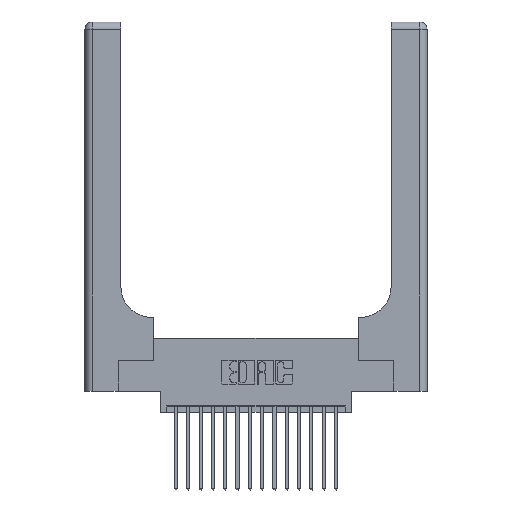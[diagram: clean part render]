
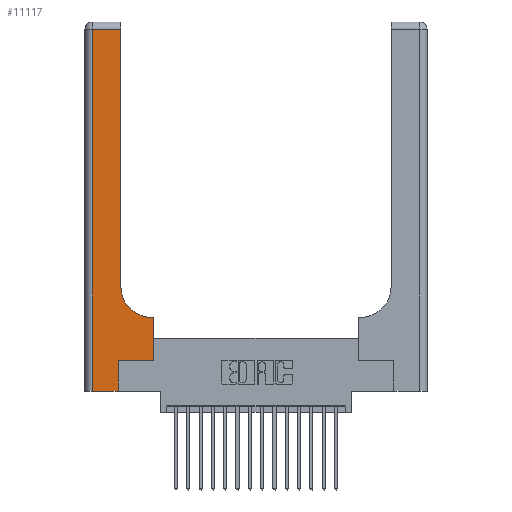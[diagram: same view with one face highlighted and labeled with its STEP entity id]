
A CAD part, top view. The second image highlights one B-rep face of the part: STEP entity #11117.
In plain terms, the highlighted planar face has unit normal (0, 0, 1).
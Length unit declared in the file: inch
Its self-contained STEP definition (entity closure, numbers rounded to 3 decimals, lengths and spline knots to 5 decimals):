
#54 = VERTEX_POINT ( 'NONE', #4918 ) ;
#96 = FACE_OUTER_BOUND ( 'NONE', #17173, .T. ) ;
#598 = EDGE_CURVE ( 'NONE', #54, #19124, #6950, .T. ) ;
#645 = VERTEX_POINT ( 'NONE', #6051 ) ;
#664 = DIRECTION ( 'NONE',  ( 0., 0., -1. ) ) ;
#934 = DIRECTION ( 'NONE',  ( 0., 1., 0. ) ) ;
#970 = CARTESIAN_POINT ( 'NONE',  ( 0.2915, 0.85, 0.37 ) ) ;
#1197 = AXIS2_PLACEMENT_3D ( 'NONE', #2160, #2093, #6903 ) ;
#1500 = EDGE_CURVE ( 'NONE', #9189, #645, #11006, .T. ) ;
#1650 = ORIENTED_EDGE ( 'NONE', *, *, #1500, .T. ) ;
#1784 = VECTOR ( 'NONE', #934, 39.37008 ) ;
#2070 = DIRECTION ( 'NONE',  ( 1., 0., 0. ) ) ;
#2093 = DIRECTION ( 'NONE',  ( 0., 0., -1. ) ) ;
#2098 = CARTESIAN_POINT ( 'NONE',  ( 0.5585, 0.6, 0.37 ) ) ;
#2117 = ORIENTED_EDGE ( 'NONE', *, *, #598, .T. ) ;
#2158 = CARTESIAN_POINT ( 'NONE',  ( 0.5415, 0.6, 0.37 ) ) ;
#2160 = CARTESIAN_POINT ( 'NONE',  ( 0., 3., 0.37 ) ) ;
#3126 = DIRECTION ( 'NONE',  ( 0., -1., 0. ) ) ;
#3160 = EDGE_CURVE ( 'NONE', #4082, #8179, #15059, .T. ) ;
#3436 = ORIENTED_EDGE ( 'NONE', *, *, #4654, .T. ) ;
#3480 = CARTESIAN_POINT ( 'NONE',  ( 0., 0., 0.37 ) ) ;
#3906 = CARTESIAN_POINT ( 'NONE',  ( 0.269, 0., 0.37 ) ) ;
#4082 = VERTEX_POINT ( 'NONE', #5858 ) ;
#4115 = ORIENTED_EDGE ( 'NONE', *, *, #7988, .T. ) ;
#4146 = VECTOR ( 'NONE', #7611, 39.37008 ) ;
#4654 = EDGE_CURVE ( 'NONE', #8179, #9564, #12822, .T. ) ;
#4918 = CARTESIAN_POINT ( 'NONE',  ( 0.06, 2.94, 0.37 ) ) ;
#5146 = LINE ( 'NONE', #15826, #12394 ) ;
#5154 = CARTESIAN_POINT ( 'NONE',  ( 0.269, 0., 0.37 ) ) ;
#5331 = DIRECTION ( 'NONE',  ( 1., 0., 0. ) ) ;
#5505 = EDGE_CURVE ( 'NONE', #9564, #8088, #5146, .T. ) ;
#5624 = CARTESIAN_POINT ( 'NONE',  ( 0.5585, 0.25, 0.37 ) ) ;
#5858 = CARTESIAN_POINT ( 'NONE',  ( 0.269, 0.25, 0.37 ) ) ;
#6051 = CARTESIAN_POINT ( 'NONE',  ( 0.2915, 2.94, 0.37 ) ) ;
#6265 = VECTOR ( 'NONE', #17879, 39.37008 ) ;
#6528 = DIRECTION ( 'NONE',  ( 0., 1., 0. ) ) ;
#6620 = ORIENTED_EDGE ( 'NONE', *, *, #17265, .T. ) ;
#6886 = CARTESIAN_POINT ( 'NONE',  ( 0., 2.94, 0.37 ) ) ;
#6903 = DIRECTION ( 'NONE',  ( -1., 0., 0. ) ) ;
#6902 = CARTESIAN_POINT ( 'NONE',  ( 0.06, 0., 0.37 ) ) ;
#6950 = LINE ( 'NONE', #15550, #8395 ) ;
#7611 = DIRECTION ( 'NONE',  ( 1., 0., 0. ) ) ;
#7811 = CARTESIAN_POINT ( 'NONE',  ( 0.269, 0.25, 0.37 ) ) ;
#7988 = EDGE_CURVE ( 'NONE', #8088, #9189, #13088, .T. ) ;
#8088 = VERTEX_POINT ( 'NONE', #2158 ) ;
#8107 = DIRECTION ( 'NONE',  ( -1., 0., 0. ) ) ;
#8179 = VERTEX_POINT ( 'NONE', #13360 ) ;
#8395 = VECTOR ( 'NONE', #3126, 39.37008 ) ;
#9189 = VERTEX_POINT ( 'NONE', #970 ) ;
#9337 = VERTEX_POINT ( 'NONE', #5154 ) ;
#9564 = VERTEX_POINT ( 'NONE', #2098 ) ;
#9720 = ORIENTED_EDGE ( 'NONE', *, *, #3160, .T. ) ;
#9775 = CARTESIAN_POINT ( 'NONE',  ( 0.2915, 3., 0.37 ) ) ;
#9946 = VECTOR ( 'NONE', #15972, 39.37008 ) ;
#10038 = VECTOR ( 'NONE', #6528, 39.37008 ) ;
#10067 = CARTESIAN_POINT ( 'NONE',  ( 0.5415, 0.85, 0.37 ) ) ;
#11006 = LINE ( 'NONE', #9775, #10038 ) ;
#11117 = ADVANCED_FACE ( 'NONE', ( #96 ), #15988, .F. ) ;
#11317 = VECTOR ( 'NONE', #2070, 39.37008 ) ;
#11649 = EDGE_CURVE ( 'NONE', #9337, #4082, #14856, .T. ) ;
#12394 = VECTOR ( 'NONE', #8107, 39.37008 ) ;
#12822 = LINE ( 'NONE', #5624, #6265 ) ;
#13088 = CIRCLE ( 'NONE', #16604, 0.25 ) ;
#13360 = CARTESIAN_POINT ( 'NONE',  ( 0.5585, 0.25, 0.37 ) ) ;
#14179 = ORIENTED_EDGE ( 'NONE', *, *, #5505, .T. ) ;
#14856 = LINE ( 'NONE', #3906, #1784 ) ;
#15059 = LINE ( 'NONE', #7811, #4146 ) ;
#15277 = EDGE_CURVE ( 'NONE', #645, #54, #18703, .T. ) ;
#15550 = CARTESIAN_POINT ( 'NONE',  ( 0.06, 3., 0.37 ) ) ;
#15826 = CARTESIAN_POINT ( 'NONE',  ( 0.2915, 0.6, 0.37 ) ) ;
#15972 = DIRECTION ( 'NONE',  ( -1., 0., 0. ) ) ;
#15988 = PLANE ( 'NONE',  #1197 ) ;
#16604 = AXIS2_PLACEMENT_3D ( 'NONE', #10067, #664, #5331 ) ;
#17067 = ORIENTED_EDGE ( 'NONE', *, *, #11649, .T. ) ;
#17173 = EDGE_LOOP ( 'NONE', ( #1650, #17549, #2117, #6620, #17067, #9720, #3436, #14179, #4115 ) ) ;
#17265 = EDGE_CURVE ( 'NONE', #19124, #9337, #20078, .T. ) ;
#17549 = ORIENTED_EDGE ( 'NONE', *, *, #15277, .T. ) ;
#17879 = DIRECTION ( 'NONE',  ( 0., 1., 0. ) ) ;
#18703 = LINE ( 'NONE', #6886, #9946 ) ;
#19124 = VERTEX_POINT ( 'NONE', #6902 ) ;
#20078 = LINE ( 'NONE', #3480, #11317 ) ;
